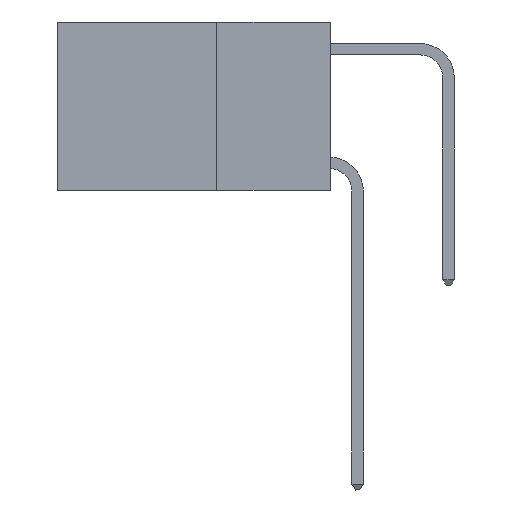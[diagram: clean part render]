
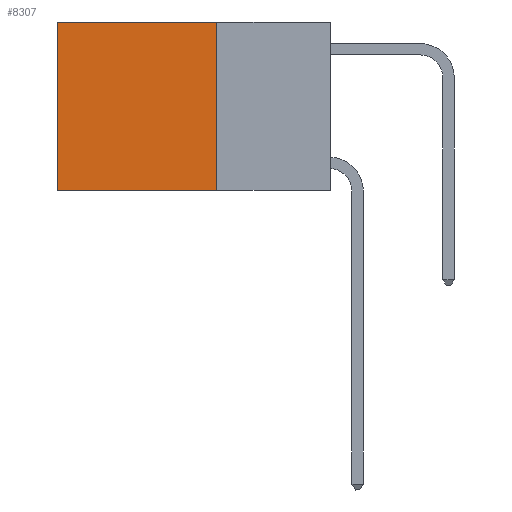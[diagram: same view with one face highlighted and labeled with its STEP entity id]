
A CAD part, left-side view. The second image highlights one B-rep face of the part: STEP entity #8307.
In plain terms, the highlighted planar face has unit normal (-1, 0, 0).
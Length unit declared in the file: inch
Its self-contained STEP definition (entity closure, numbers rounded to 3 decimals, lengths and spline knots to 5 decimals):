
#255 = CARTESIAN_POINT ( 'NONE',  ( 0.2625, 0.25, -0.37 ) ) ;
#579 = DIRECTION ( 'NONE',  ( 1., 0., 0. ) ) ;
#1139 = VERTEX_POINT ( 'NONE', #23857 ) ;
#2681 = LINE ( 'NONE', #8105, #14317 ) ;
#3336 = ORIENTED_EDGE ( 'NONE', *, *, #25181, .T. ) ;
#3514 = VECTOR ( 'NONE', #23030, 39.37008 ) ;
#4576 = ORIENTED_EDGE ( 'NONE', *, *, #5089, .F. ) ;
#4610 = ORIENTED_EDGE ( 'NONE', *, *, #14150, .F. ) ;
#4754 = EDGE_LOOP ( 'NONE', ( #13822, #4576, #4610, #3336 ) ) ;
#5089 = EDGE_CURVE ( 'NONE', #17446, #28968, #2681, .T. ) ;
#6655 = DIRECTION ( 'NONE',  ( 0., 0., -1. ) ) ;
#7944 = VECTOR ( 'NONE', #6655, 39.37008 ) ;
#8105 = CARTESIAN_POINT ( 'NONE',  ( 0.2625, 0.25, -0.37 ) ) ;
#8307 = ADVANCED_FACE ( 'NONE', ( #22024 ), #23715, .F. ) ;
#9003 = CARTESIAN_POINT ( 'NONE',  ( 0.2625, 0.25, 0. ) ) ;
#9761 = LINE ( 'NONE', #18351, #3514 ) ;
#12760 = DIRECTION ( 'NONE',  ( 0., 1., 0. ) ) ;
#13329 = DIRECTION ( 'NONE',  ( 0., 1., 0. ) ) ;
#13822 = ORIENTED_EDGE ( 'NONE', *, *, #25328, .T. ) ;
#14150 = EDGE_CURVE ( 'NONE', #27155, #17446, #20192, .T. ) ;
#14317 = VECTOR ( 'NONE', #12760, 39.37008 ) ;
#16816 = CARTESIAN_POINT ( 'NONE',  ( 0.2625, 0.6, -0.37 ) ) ;
#16866 = DIRECTION ( 'NONE',  ( 0., 0., -1. ) ) ;
#17446 = VERTEX_POINT ( 'NONE', #255 ) ;
#18351 = CARTESIAN_POINT ( 'NONE',  ( 0.2625, 0.6, 0. ) ) ;
#20192 = LINE ( 'NONE', #9003, #7944 ) ;
#20550 = AXIS2_PLACEMENT_3D ( 'NONE', #26042, #579, #16866 ) ;
#22024 = FACE_OUTER_BOUND ( 'NONE', #4754, .T. ) ;
#23030 = DIRECTION ( 'NONE',  ( 0., 0., -1. ) ) ;
#23034 = CARTESIAN_POINT ( 'NONE',  ( 0.2625, 0.25, 0. ) ) ;
#23715 = PLANE ( 'NONE',  #20550 ) ;
#23857 = CARTESIAN_POINT ( 'NONE',  ( 0.2625, 0.6, 0. ) ) ;
#25181 = EDGE_CURVE ( 'NONE', #27155, #1139, #27028, .T. ) ;
#25328 = EDGE_CURVE ( 'NONE', #1139, #28968, #9761, .T. ) ;
#25628 = VECTOR ( 'NONE', #13329, 39.37008 ) ;
#26042 = CARTESIAN_POINT ( 'NONE',  ( 0.2625, 0.25, 0. ) ) ;
#27028 = LINE ( 'NONE', #27117, #25628 ) ;
#27117 = CARTESIAN_POINT ( 'NONE',  ( 0.2625, 0.25, 0. ) ) ;
#27155 = VERTEX_POINT ( 'NONE', #23034 ) ;
#28968 = VERTEX_POINT ( 'NONE', #16816 ) ;
